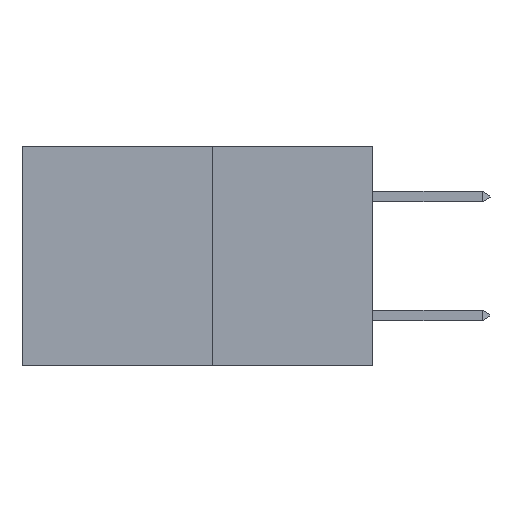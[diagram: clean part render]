
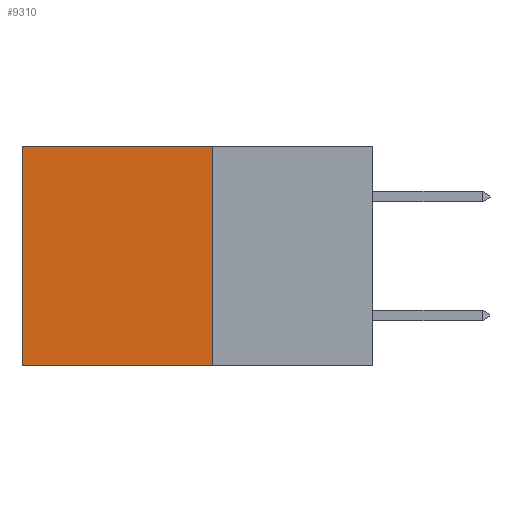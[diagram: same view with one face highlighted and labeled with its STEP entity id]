
A CAD part, left-side view. The second image highlights one B-rep face of the part: STEP entity #9310.
In plain terms, the highlighted planar face has unit normal (-1, 0, 0).
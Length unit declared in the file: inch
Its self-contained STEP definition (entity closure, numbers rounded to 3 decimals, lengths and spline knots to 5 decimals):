
#700 = VERTEX_POINT ( 'NONE', #1747 ) ;
#1461 = DIRECTION ( 'NONE',  ( 0., 0., -1. ) ) ;
#1747 = CARTESIAN_POINT ( 'NONE',  ( 0.277, 0.27, 0. ) ) ;
#1872 = CARTESIAN_POINT ( 'NONE',  ( 0.277, 0.27, -0.37 ) ) ;
#2151 = CARTESIAN_POINT ( 'NONE',  ( 0.277, 0.59, 0. ) ) ;
#2267 = LINE ( 'NONE', #8861, #8263 ) ;
#2422 = ORIENTED_EDGE ( 'NONE', *, *, #6887, .T. ) ;
#2602 = EDGE_CURVE ( 'NONE', #700, #4643, #2267, .T. ) ;
#2918 = ORIENTED_EDGE ( 'NONE', *, *, #2602, .F. ) ;
#3776 = ORIENTED_EDGE ( 'NONE', *, *, #9690, .F. ) ;
#3876 = PLANE ( 'NONE',  #4631 ) ;
#3889 = CARTESIAN_POINT ( 'NONE',  ( 0.277, 0.27, 0. ) ) ;
#4290 = ORIENTED_EDGE ( 'NONE', *, *, #4939, .T. ) ;
#4303 = DIRECTION ( 'NONE',  ( 0., 1., 0. ) ) ;
#4631 = AXIS2_PLACEMENT_3D ( 'NONE', #5393, #6192, #1461 ) ;
#4643 = VERTEX_POINT ( 'NONE', #6516 ) ;
#4908 = DIRECTION ( 'NONE',  ( 0., 0., -1. ) ) ;
#4939 = EDGE_CURVE ( 'NONE', #9887, #9276, #7364, .T. ) ;
#5023 = CARTESIAN_POINT ( 'NONE',  ( 0.277, 0.59, -0.37 ) ) ;
#5393 = CARTESIAN_POINT ( 'NONE',  ( 0.277, 0.27, -0.37 ) ) ;
#6192 = DIRECTION ( 'NONE',  ( 1., 0., 0. ) ) ;
#6349 = LINE ( 'NONE', #1872, #8181 ) ;
#6516 = CARTESIAN_POINT ( 'NONE',  ( 0.277, 0.27, -0.37 ) ) ;
#6887 = EDGE_CURVE ( 'NONE', #700, #9887, #9010, .T. ) ;
#6915 = CARTESIAN_POINT ( 'NONE',  ( 0.277, 0.59, -0.37 ) ) ;
#7364 = LINE ( 'NONE', #5023, #8930 ) ;
#7831 = EDGE_LOOP ( 'NONE', ( #4290, #3776, #2918, #2422 ) ) ;
#8181 = VECTOR ( 'NONE', #4303, 39.37008 ) ;
#8263 = VECTOR ( 'NONE', #9103, 39.37008 ) ;
#8522 = DIRECTION ( 'NONE',  ( 0., 1., 0. ) ) ;
#8780 = VECTOR ( 'NONE', #8522, 39.37008 ) ;
#8861 = CARTESIAN_POINT ( 'NONE',  ( 0.277, 0.27, -0.37 ) ) ;
#8930 = VECTOR ( 'NONE', #4908, 39.37008 ) ;
#9010 = LINE ( 'NONE', #3889, #8780 ) ;
#9103 = DIRECTION ( 'NONE',  ( 0., 0., -1. ) ) ;
#9274 = FACE_OUTER_BOUND ( 'NONE', #7831, .T. ) ;
#9276 = VERTEX_POINT ( 'NONE', #6915 ) ;
#9310 = ADVANCED_FACE ( 'NONE', ( #9274 ), #3876, .F. ) ;
#9690 = EDGE_CURVE ( 'NONE', #4643, #9276, #6349, .T. ) ;
#9887 = VERTEX_POINT ( 'NONE', #2151 ) ;
